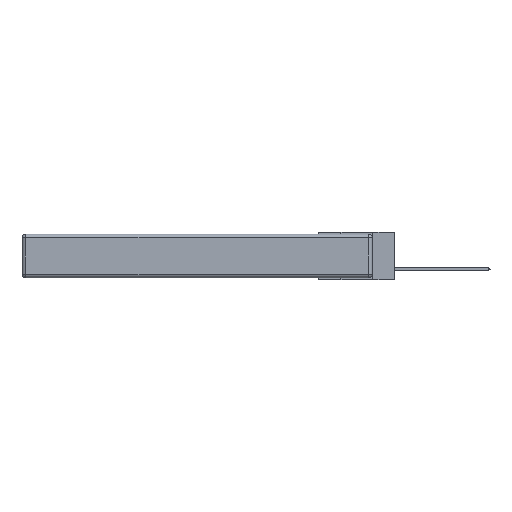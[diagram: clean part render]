
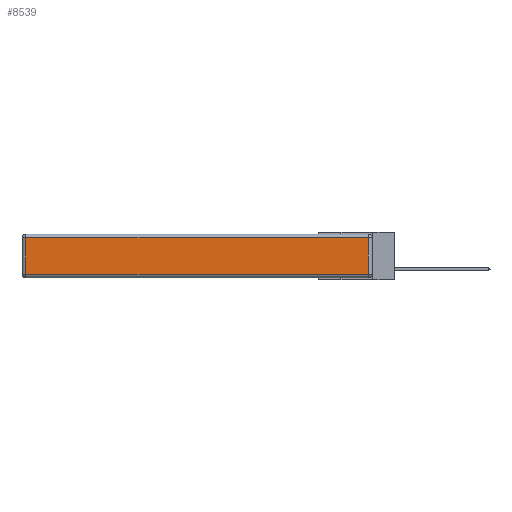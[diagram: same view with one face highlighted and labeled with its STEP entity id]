
A CAD part, left-side view. The second image highlights one B-rep face of the part: STEP entity #8539.
In plain terms, the highlighted planar face has unit normal (-1, 0, 0).
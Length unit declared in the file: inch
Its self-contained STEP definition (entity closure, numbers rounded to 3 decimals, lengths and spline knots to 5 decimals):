
#651 = LINE ( 'NONE', #9532, #14267 ) ;
#1404 = ORIENTED_EDGE ( 'NONE', *, *, #3008, .T. ) ;
#1510 = VECTOR ( 'NONE', #11965, 39.37008 ) ;
#1784 = CARTESIAN_POINT ( 'NONE',  ( 0., 0., -0.343 ) ) ;
#2565 = AXIS2_PLACEMENT_3D ( 'NONE', #1784, #13971, #5098 ) ;
#2856 = ORIENTED_EDGE ( 'NONE', *, *, #8029, .T. ) ;
#3008 = EDGE_CURVE ( 'NONE', #14294, #12917, #8683, .T. ) ;
#3070 = ORIENTED_EDGE ( 'NONE', *, *, #12294, .T. ) ;
#3688 = CARTESIAN_POINT ( 'NONE',  ( 0., 2.75, -0.03 ) ) ;
#4442 = CARTESIAN_POINT ( 'NONE',  ( 0., 2.72, -0.03 ) ) ;
#4706 = VECTOR ( 'NONE', #9238, 39.37008 ) ;
#5098 = DIRECTION ( 'NONE',  ( 0., 0., 1. ) ) ;
#5311 = CARTESIAN_POINT ( 'NONE',  ( 0., 0.03, -0.343 ) ) ;
#5437 = EDGE_CURVE ( 'NONE', #6742, #8308, #11024, .T. ) ;
#5950 = CARTESIAN_POINT ( 'NONE',  ( 0., 0.03, -0.313 ) ) ;
#6742 = VERTEX_POINT ( 'NONE', #11487 ) ;
#8029 = EDGE_CURVE ( 'NONE', #12917, #6742, #651, .T. ) ;
#8308 = VERTEX_POINT ( 'NONE', #5950 ) ;
#8339 = LINE ( 'NONE', #5311, #8843 ) ;
#8539 = ADVANCED_FACE ( 'NONE', ( #13069 ), #9514, .T. ) ;
#8663 = CARTESIAN_POINT ( 'NONE',  ( 0., 0.03, -0.03 ) ) ;
#8683 = LINE ( 'NONE', #3688, #4706 ) ;
#8843 = VECTOR ( 'NONE', #11484, 39.37008 ) ;
#9238 = DIRECTION ( 'NONE',  ( 0., 1., 0. ) ) ;
#9514 = PLANE ( 'NONE',  #2565 ) ;
#9532 = CARTESIAN_POINT ( 'NONE',  ( 0., 2.72, -0.343 ) ) ;
#10550 = EDGE_LOOP ( 'NONE', ( #14005, #3070, #1404, #2856 ) ) ;
#10758 = CARTESIAN_POINT ( 'NONE',  ( 0., 0., -0.313 ) ) ;
#11024 = LINE ( 'NONE', #10758, #1510 ) ;
#11484 = DIRECTION ( 'NONE',  ( 0., 0., 1. ) ) ;
#11487 = CARTESIAN_POINT ( 'NONE',  ( 0., 2.72, -0.313 ) ) ;
#11726 = DIRECTION ( 'NONE',  ( 0., 0., -1. ) ) ;
#11965 = DIRECTION ( 'NONE',  ( 0., -1., 0. ) ) ;
#12294 = EDGE_CURVE ( 'NONE', #8308, #14294, #8339, .T. ) ;
#12917 = VERTEX_POINT ( 'NONE', #4442 ) ;
#13069 = FACE_OUTER_BOUND ( 'NONE', #10550, .T. ) ;
#13971 = DIRECTION ( 'NONE',  ( -1., 0., 0. ) ) ;
#14005 = ORIENTED_EDGE ( 'NONE', *, *, #5437, .T. ) ;
#14267 = VECTOR ( 'NONE', #11726, 39.37008 ) ;
#14294 = VERTEX_POINT ( 'NONE', #8663 ) ;
